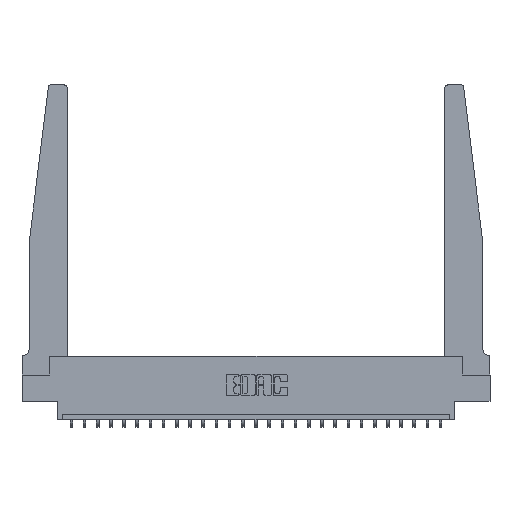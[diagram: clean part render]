
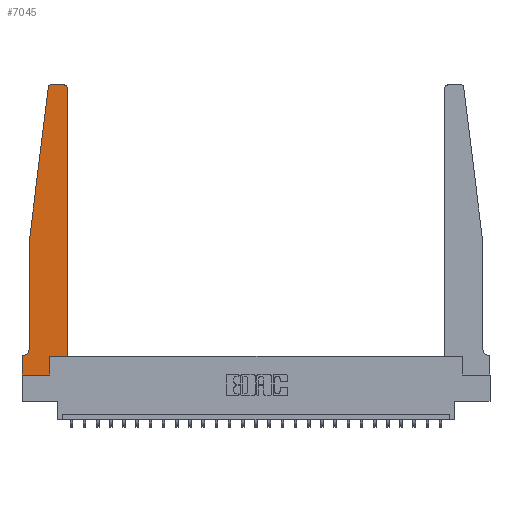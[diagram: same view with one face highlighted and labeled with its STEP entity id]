
A CAD part, top view. The second image highlights one B-rep face of the part: STEP entity #7045.
In plain terms, the highlighted planar face has unit normal (0, 0, 1).
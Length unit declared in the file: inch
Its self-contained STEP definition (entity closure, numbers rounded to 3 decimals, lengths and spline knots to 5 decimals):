
#763 = EDGE_CURVE ( 'NONE', #19604, #3298, #7692, .T. ) ;
#914 = VECTOR ( 'NONE', #1132, 39.37008 ) ;
#1132 = DIRECTION ( 'NONE',  ( 1., 0., 0. ) ) ;
#1149 = ORIENTED_EDGE ( 'NONE', *, *, #2295, .T. ) ;
#1428 = DIRECTION ( 'NONE',  ( -0.122, -0.992, 0. ) ) ;
#1499 = ORIENTED_EDGE ( 'NONE', *, *, #12040, .T. ) ;
#1833 = CARTESIAN_POINT ( 'NONE',  ( 0., 0.1875, 0.37 ) ) ;
#2083 = DIRECTION ( 'NONE',  ( 0., 1., 0. ) ) ;
#2171 = CARTESIAN_POINT ( 'NONE',  ( 0., 0.1875, 0.37 ) ) ;
#2233 = EDGE_CURVE ( 'NONE', #8705, #13197, #12062, .T. ) ;
#2234 = EDGE_CURVE ( 'NONE', #13825, #15106, #17048, .T. ) ;
#2255 = PLANE ( 'NONE',  #9305 ) ;
#2295 = EDGE_CURVE ( 'NONE', #3298, #16839, #11479, .T. ) ;
#3044 = ORIENTED_EDGE ( 'NONE', *, *, #8084, .T. ) ;
#3175 = CARTESIAN_POINT ( 'NONE',  ( 0.065, 0.2375, 0.37 ) ) ;
#3246 = DIRECTION ( 'NONE',  ( 0., 0., -1. ) ) ;
#3298 = VERTEX_POINT ( 'NONE', #6769 ) ;
#3323 = ORIENTED_EDGE ( 'NONE', *, *, #14774, .T. ) ;
#3389 = CARTESIAN_POINT ( 'NONE',  ( 0.2605, 0., 0.37 ) ) ;
#4027 = VECTOR ( 'NONE', #2083, 39.37008 ) ;
#4053 = CARTESIAN_POINT ( 'NONE',  ( 0.2605, 0.18, 0.37 ) ) ;
#4233 = DIRECTION ( 'NONE',  ( 1., 0., 0. ) ) ;
#4722 = EDGE_CURVE ( 'NONE', #23530, #18736, #10186, .T. ) ;
#4969 = LINE ( 'NONE', #12895, #18836 ) ;
#5398 = DIRECTION ( 'NONE',  ( -1., 0., 0. ) ) ;
#6102 = ORIENTED_EDGE ( 'NONE', *, *, #11808, .T. ) ;
#6111 = EDGE_CURVE ( 'NONE', #22597, #13825, #23325, .T. ) ;
#6420 = CARTESIAN_POINT ( 'NONE',  ( 0.425, 0.18, 0.37 ) ) ;
#6438 = VECTOR ( 'NONE', #1428, 39.37008 ) ;
#6548 = CARTESIAN_POINT ( 'NONE',  ( 0.425, 2.72, 0.37 ) ) ;
#6769 = CARTESIAN_POINT ( 'NONE',  ( 0.24675, 2.72367, 0.37 ) ) ;
#6782 = CARTESIAN_POINT ( 'NONE',  ( 0., 0., 0.37 ) ) ;
#7045 = ADVANCED_FACE ( 'NONE', ( #13832 ), #2255, .T. ) ;
#7158 = CARTESIAN_POINT ( 'NONE',  ( 0.395, 2.72, 0.37 ) ) ;
#7692 = CIRCLE ( 'NONE', #11576, 0.03 ) ;
#8084 = EDGE_CURVE ( 'NONE', #18736, #11321, #11200, .T. ) ;
#8282 = VECTOR ( 'NONE', #12427, 39.37008 ) ;
#8438 = ORIENTED_EDGE ( 'NONE', *, *, #9179, .T. ) ;
#8705 = VERTEX_POINT ( 'NONE', #3175 ) ;
#9075 = DIRECTION ( 'NONE',  ( 1., 0., 0. ) ) ;
#9120 = VECTOR ( 'NONE', #5398, 39.37008 ) ;
#9179 = EDGE_CURVE ( 'NONE', #15106, #19604, #12023, .T. ) ;
#9305 = AXIS2_PLACEMENT_3D ( 'NONE', #2171, #15567, #4233 ) ;
#9328 = DIRECTION ( 'NONE',  ( 0., 0., 1. ) ) ;
#10186 = LINE ( 'NONE', #6782, #20171 ) ;
#10801 = EDGE_LOOP ( 'NONE', ( #8438, #14909, #1149, #3323, #20830, #17007, #18763, #3044, #1499, #6102, #15525, #11166 ) ) ;
#11166 = ORIENTED_EDGE ( 'NONE', *, *, #2234, .T. ) ;
#11200 = LINE ( 'NONE', #14506, #914 ) ;
#11321 = VERTEX_POINT ( 'NONE', #3389 ) ;
#11352 = VERTEX_POINT ( 'NONE', #17174 ) ;
#11479 = LINE ( 'NONE', #20418, #6438 ) ;
#11576 = AXIS2_PLACEMENT_3D ( 'NONE', #18629, #9328, #16224 ) ;
#11808 = EDGE_CURVE ( 'NONE', #11352, #22597, #4969, .T. ) ;
#12023 = LINE ( 'NONE', #23390, #22011 ) ;
#12040 = EDGE_CURVE ( 'NONE', #11321, #11352, #24187, .T. ) ;
#12062 = CIRCLE ( 'NONE', #16318, 0.05 ) ;
#12427 = DIRECTION ( 'NONE',  ( 0., 1., 0. ) ) ;
#12509 = EDGE_CURVE ( 'NONE', #13197, #23530, #14685, .T. ) ;
#12895 = CARTESIAN_POINT ( 'NONE',  ( 0.425, 0.18, 0.37 ) ) ;
#13197 = VERTEX_POINT ( 'NONE', #13998 ) ;
#13745 = VECTOR ( 'NONE', #20595, 39.37008 ) ;
#13825 = VERTEX_POINT ( 'NONE', #6548 ) ;
#13832 = FACE_OUTER_BOUND ( 'NONE', #10801, .T. ) ;
#13998 = CARTESIAN_POINT ( 'NONE',  ( 0.015, 0.1875, 0.37 ) ) ;
#14506 = CARTESIAN_POINT ( 'NONE',  ( 0., 0., 0.37 ) ) ;
#14631 = CARTESIAN_POINT ( 'NONE',  ( 0.015, 0.2375, 0.37 ) ) ;
#14685 = LINE ( 'NONE', #20504, #9120 ) ;
#14774 = EDGE_CURVE ( 'NONE', #16839, #8705, #18982, .T. ) ;
#14830 = CARTESIAN_POINT ( 'NONE',  ( 0., 0., 0.37 ) ) ;
#14909 = ORIENTED_EDGE ( 'NONE', *, *, #763, .T. ) ;
#15106 = VERTEX_POINT ( 'NONE', #17761 ) ;
#15525 = ORIENTED_EDGE ( 'NONE', *, *, #6111, .T. ) ;
#15567 = DIRECTION ( 'NONE',  ( 0., 0., 1. ) ) ;
#15695 = CARTESIAN_POINT ( 'NONE',  ( 0.27653, 2.75, 0.37 ) ) ;
#15867 = DIRECTION ( 'NONE',  ( -1., 0., 0. ) ) ;
#16224 = DIRECTION ( 'NONE',  ( 1., 0., 0. ) ) ;
#16318 = AXIS2_PLACEMENT_3D ( 'NONE', #14631, #3246, #16543 ) ;
#16543 = DIRECTION ( 'NONE',  ( -1., 0., 0. ) ) ;
#16839 = VERTEX_POINT ( 'NONE', #20354 ) ;
#17007 = ORIENTED_EDGE ( 'NONE', *, *, #12509, .T. ) ;
#17048 = CIRCLE ( 'NONE', #21372, 0.03 ) ;
#17174 = CARTESIAN_POINT ( 'NONE',  ( 0.2605, 0.18, 0.37 ) ) ;
#17761 = CARTESIAN_POINT ( 'NONE',  ( 0.395, 2.75, 0.37 ) ) ;
#18629 = CARTESIAN_POINT ( 'NONE',  ( 0.27653, 2.72, 0.37 ) ) ;
#18684 = CARTESIAN_POINT ( 'NONE',  ( 0.065, 1.25, 0.37 ) ) ;
#18736 = VERTEX_POINT ( 'NONE', #14830 ) ;
#18763 = ORIENTED_EDGE ( 'NONE', *, *, #4722, .T. ) ;
#18836 = VECTOR ( 'NONE', #22266, 39.37008 ) ;
#18982 = LINE ( 'NONE', #18684, #13745 ) ;
#19604 = VERTEX_POINT ( 'NONE', #15695 ) ;
#19964 = DIRECTION ( 'NONE',  ( 0., -1., 0. ) ) ;
#20171 = VECTOR ( 'NONE', #19964, 39.37008 ) ;
#20336 = DIRECTION ( 'NONE',  ( 0., 0., 1. ) ) ;
#20354 = CARTESIAN_POINT ( 'NONE',  ( 0.065, 1.25, 0.37 ) ) ;
#20418 = CARTESIAN_POINT ( 'NONE',  ( 0.065, 1.25, 0.37 ) ) ;
#20504 = CARTESIAN_POINT ( 'NONE',  ( 0.065, 0.1875, 0.37 ) ) ;
#20595 = DIRECTION ( 'NONE',  ( 0., -1., 0. ) ) ;
#20830 = ORIENTED_EDGE ( 'NONE', *, *, #2233, .T. ) ;
#21372 = AXIS2_PLACEMENT_3D ( 'NONE', #7158, #20336, #9075 ) ;
#21803 = CARTESIAN_POINT ( 'NONE',  ( 0.425, 0.18, 0.37 ) ) ;
#22011 = VECTOR ( 'NONE', #15867, 39.37008 ) ;
#22266 = DIRECTION ( 'NONE',  ( 1., 0., 0. ) ) ;
#22597 = VERTEX_POINT ( 'NONE', #6420 ) ;
#23325 = LINE ( 'NONE', #21803, #8282 ) ;
#23390 = CARTESIAN_POINT ( 'NONE',  ( 0.25, 2.75, 0.37 ) ) ;
#23530 = VERTEX_POINT ( 'NONE', #1833 ) ;
#24187 = LINE ( 'NONE', #4053, #4027 ) ;
